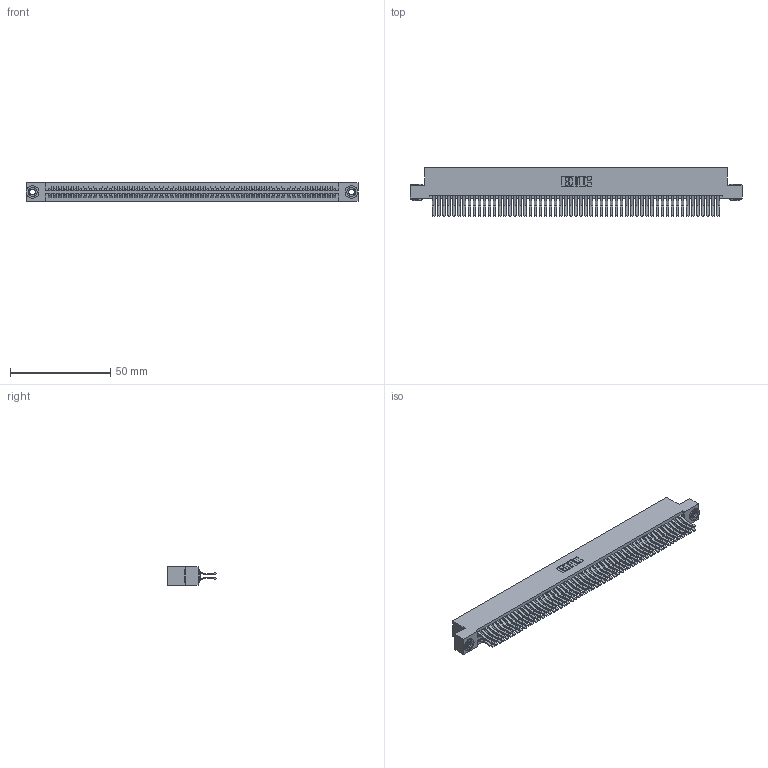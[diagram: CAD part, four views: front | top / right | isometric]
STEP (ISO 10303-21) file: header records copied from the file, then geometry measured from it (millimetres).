
FILE_DESCRIPTION (( 'STEP AP203' ), '1' );
FILE_NAME ('395-114-560-203.STEP', '2018-12-01T20:19:20', ( '' ), ( '' ), 'SwSTEP 2.0', 'SolidWorks 2016', '' );
FILE_SCHEMA (( 'CONFIG_CONTROL_DESIGN' ));
Length unit declared in the file: inch
Products named in the file (4): 345-292-001_560 Tail; 345-250-002_345-250-002-102; 395-114-560-203; 345 Part_Flush Mounting Lugs - 0.156 Dia-TH
Assembly tree (117 placements, depth 2):
  395-114-560-203
    345 Part_Flush Mounting Lugs - 0.156 Dia-TH
    345-292-001_560 Tail  x114
    345-250-002_345-250-002-102  x2
Bounding box: 165.99 x 24.45 x 9.4 mm (x, y, z)
Volume: 17030.2 mm3; surface area: 27590.7 mm2
Topology: 117 solids, 117 shells, 6092 faces, 18087 edges, 11902 vertices
Faces by surface type: plane 3852, cylinder 2232, cone 8
Entity records: 43442 total; most frequent: CARTESIAN_POINT 7243, ORIENTED_EDGE 7170, DIRECTION 6403, EDGE_CURVE 3585, LINE 3197, VECTOR 3197, VERTEX_POINT 2386, AXIS2_PLACEMENT_3D 1603
